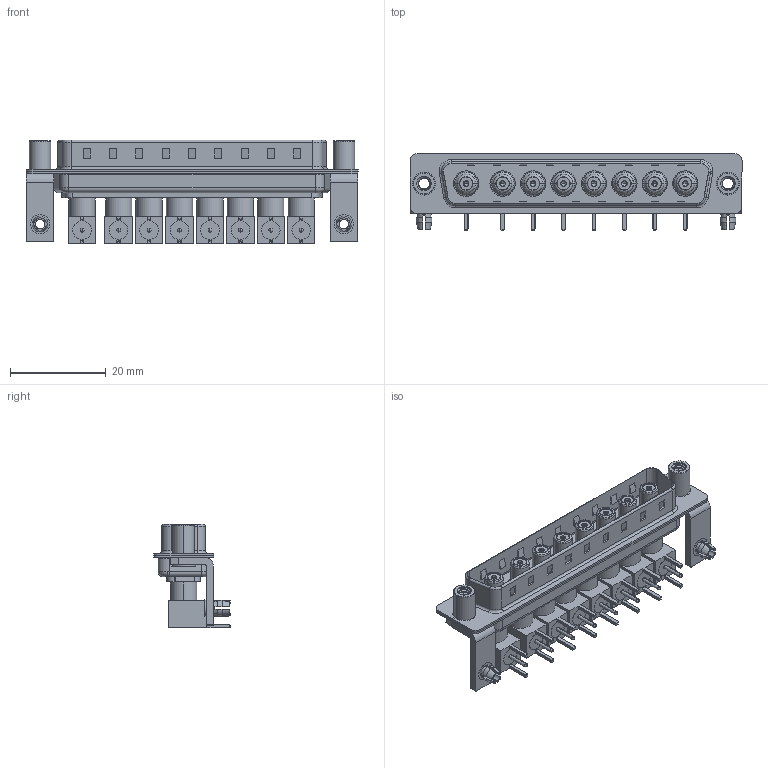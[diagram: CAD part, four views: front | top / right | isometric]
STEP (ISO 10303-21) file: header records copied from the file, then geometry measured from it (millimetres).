
FILE_DESCRIPTION (( 'STEP AP203' ), '1' );
FILE_NAME ('629-8W8-240-7T5.STEP', '2022-05-14T06:19:46', ( '' ), ( '' ), 'SwSTEP 2.0', 'SolidWorks 2020', '' );
FILE_SCHEMA (( 'CONFIG_CONTROL_DESIGN' ));
Length unit declared in the file: millimetre
Products named in the file (22): Co-Ax Jack_RA PC Tail; 629Combo Housing_8W8; Co-Ax Jack Assy_RA; Locking Collar; 629Combo Board Lock; 629Combo Shell Rear_37 Contacts; 629Combo Shell Front_37 Contacts; Insulator Socket 2; 629-8W8-240-7T5; 629Combo Threaded Standoff_5; Insulator Socket; Insulator RA Pin; 629Combo Stabilizer Bracket; Socket_RA; RA Back Shell
Assembly tree (73 placements, depth 3):
  629-8W8-240-7T5
    629Combo Housing_8W8
    629Combo Shell Rear_37 Contacts
    629Combo Shell Front_37 Contacts
    629Combo Stabilizer Bracket  x2
    629Combo Board Lock  x2
    629Combo Threaded Standoff_5  x2
    Co-Ax Jack Assy_RA
      Co-Ax Jack_RA PC Tail
      Insulator Socket
      Insulator Socket 2
      Locking Collar
      Socket_RA
      RA Back Shell
      Insulator RA Pin
    Co-Ax Jack Assy_RA
      Co-Ax Jack_RA PC Tail
      Insulator Socket
      Insulator Socket 2
      Locking Collar
      Socket_RA
      RA Back Shell
      Insulator RA Pin
    Co-Ax Jack Assy_RA
      Co-Ax Jack_RA PC Tail
      Insulator Socket
      Insulator Socket 2
      Locking Collar
      Socket_RA
      RA Back Shell
      Insulator RA Pin
    Co-Ax Jack Assy_RA
      Co-Ax Jack_RA PC Tail
      Insulator Socket
      Insulator Socket 2
      Locking Collar
      Socket_RA
      RA Back Shell
      Insulator RA Pin
    Co-Ax Jack Assy_RA
      Co-Ax Jack_RA PC Tail
      Insulator Socket
      Insulator Socket 2
      Locking Collar
      Socket_RA
      RA Back Shell
      Insulator RA Pin
    Co-Ax Jack Assy_RA
      Co-Ax Jack_RA PC Tail
      Insulator Socket
      Insulator Socket 2
      Locking Collar
      Socket_RA
      RA Back Shell
      Insulator RA Pin
    Co-Ax Jack Assy_RA
      Co-Ax Jack_RA PC Tail
      Insulator Socket
      Insulator Socket 2
      Locking Collar
Bounding box: 69.4 x 16 x 21.71 mm (x, y, z)
Volume: 6494.2 mm3; surface area: 17880.2 mm2
Topology: 65 solids, 65 shells, 1808 faces, 4301 edges, 2688 vertices
Faces by surface type: cylinder 769, plane 729, cone 182, torus 98, sphere 16, bspline 14
Entity records: 25632 total; most frequent: CARTESIAN_POINT 5594, DIRECTION 3599, ORIENTED_EDGE 3270, EDGE_CURVE 1635, AXIS2_PLACEMENT_3D 1333, VERTEX_POINT 1040, LINE 933, VECTOR 933
